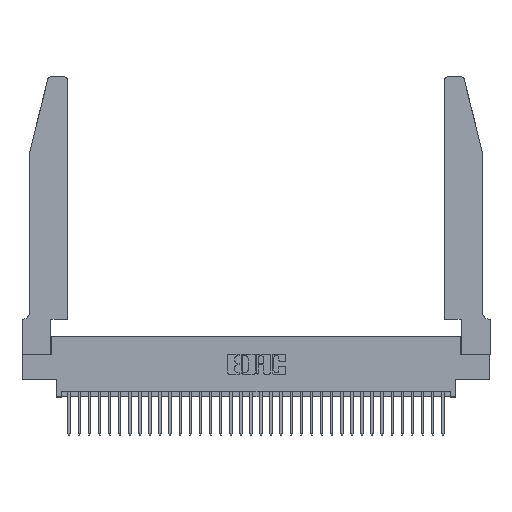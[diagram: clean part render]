
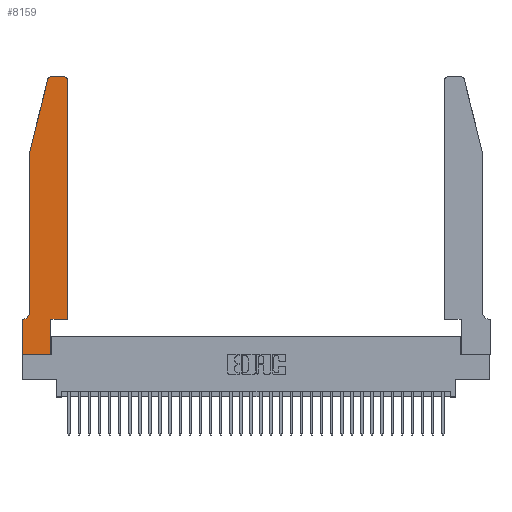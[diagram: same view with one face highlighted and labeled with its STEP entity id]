
A CAD part, top view. The second image highlights one B-rep face of the part: STEP entity #8159.
In plain terms, the highlighted planar face has unit normal (0, 0, 1).
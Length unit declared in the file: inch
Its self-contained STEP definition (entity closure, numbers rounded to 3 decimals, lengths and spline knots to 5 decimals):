
#110 = CARTESIAN_POINT ( 'NONE',  ( 0., 0., 0.37 ) ) ;
#474 = CIRCLE ( 'NONE', #28129, 0.03 ) ;
#939 = DIRECTION ( 'NONE',  ( 0., 0., 1. ) ) ;
#1340 = LINE ( 'NONE', #6033, #12000 ) ;
#2242 = EDGE_CURVE ( 'NONE', #10344, #26279, #31111, .T. ) ;
#2344 = DIRECTION ( 'NONE',  ( -1., 0., 0. ) ) ;
#3501 = VECTOR ( 'NONE', #15884, 39.37008 ) ;
#3804 = VECTOR ( 'NONE', #2344, 39.37008 ) ;
#4209 = ORIENTED_EDGE ( 'NONE', *, *, #34407, .T. ) ;
#4820 = AXIS2_PLACEMENT_3D ( 'NONE', #14662, #939, #14545 ) ;
#4962 = CARTESIAN_POINT ( 'NONE',  ( 0.4505, 0.35, 0.37 ) ) ;
#5090 = CARTESIAN_POINT ( 'NONE',  ( 0.4505, 2.72, 0.37 ) ) ;
#5333 = DIRECTION ( 'NONE',  ( 1., 0., 0. ) ) ;
#5356 = CARTESIAN_POINT ( 'NONE',  ( 0.4205, 2.75, 0.37 ) ) ;
#5872 = CARTESIAN_POINT ( 'NONE',  ( 0.284, 2.75, 0.37 ) ) ;
#6033 = CARTESIAN_POINT ( 'NONE',  ( 0.0755, 2., 0.37 ) ) ;
#6221 = VERTEX_POINT ( 'NONE', #25799 ) ;
#7044 = ORIENTED_EDGE ( 'NONE', *, *, #18117, .T. ) ;
#8021 = DIRECTION ( 'NONE',  ( 1., 0., 0. ) ) ;
#8159 = ADVANCED_FACE ( 'NONE', ( #14410 ), #26431, .T. ) ;
#8172 = VECTOR ( 'NONE', #12169, 39.37008 ) ;
#8259 = DIRECTION ( 'NONE',  ( 0., 0., -1. ) ) ;
#8478 = CARTESIAN_POINT ( 'NONE',  ( 0.4505, 0.35, 0.37 ) ) ;
#8535 = CARTESIAN_POINT ( 'NONE',  ( 0.25487, 2.72718, 0.37 ) ) ;
#9399 = VECTOR ( 'NONE', #11565, 39.37008 ) ;
#9536 = AXIS2_PLACEMENT_3D ( 'NONE', #21738, #8259, #18868 ) ;
#9808 = ORIENTED_EDGE ( 'NONE', *, *, #18643, .T. ) ;
#10032 = CARTESIAN_POINT ( 'NONE',  ( 0.0755, 2., 0.37 ) ) ;
#10326 = VECTOR ( 'NONE', #5333, 39.37008 ) ;
#10344 = VERTEX_POINT ( 'NONE', #28666 ) ;
#10536 = ORIENTED_EDGE ( 'NONE', *, *, #25302, .T. ) ;
#11201 = CARTESIAN_POINT ( 'NONE',  ( 0.2865, 0., 0.37 ) ) ;
#11354 = LINE ( 'NONE', #8478, #22037 ) ;
#11515 = DIRECTION ( 'NONE',  ( -0.239, -0.971, 0. ) ) ;
#11565 = DIRECTION ( 'NONE',  ( -1., 0., 0. ) ) ;
#11732 = VERTEX_POINT ( 'NONE', #8535 ) ;
#12000 = VECTOR ( 'NONE', #11515, 39.37008 ) ;
#12106 = EDGE_CURVE ( 'NONE', #34551, #10344, #24782, .T. ) ;
#12169 = DIRECTION ( 'NONE',  ( 0., 1., 0. ) ) ;
#12425 = EDGE_CURVE ( 'NONE', #18082, #6221, #20968, .T. ) ;
#12602 = CARTESIAN_POINT ( 'NONE',  ( 0.0755, 0.42, 0.37 ) ) ;
#13332 = LINE ( 'NONE', #10032, #3501 ) ;
#13388 = VECTOR ( 'NONE', #35286, 39.37008 ) ;
#13466 = EDGE_CURVE ( 'NONE', #31652, #23869, #15385, .T. ) ;
#14410 = FACE_OUTER_BOUND ( 'NONE', #34535, .T. ) ;
#14545 = DIRECTION ( 'NONE',  ( 1., 0., 0. ) ) ;
#14662 = CARTESIAN_POINT ( 'NONE',  ( 0.4205, 2.72, 0.37 ) ) ;
#15054 = CARTESIAN_POINT ( 'NONE',  ( 0.2865, 0.35, 0.37 ) ) ;
#15385 = LINE ( 'NONE', #18673, #3804 ) ;
#15562 = ORIENTED_EDGE ( 'NONE', *, *, #24809, .T. ) ;
#15884 = DIRECTION ( 'NONE',  ( 0., -1., 0. ) ) ;
#16419 = EDGE_CURVE ( 'NONE', #26704, #20437, #11354, .T. ) ;
#16990 = CARTESIAN_POINT ( 'NONE',  ( 0., 0.35, 0.37 ) ) ;
#17877 = ORIENTED_EDGE ( 'NONE', *, *, #18945, .T. ) ;
#18082 = VERTEX_POINT ( 'NONE', #11201 ) ;
#18117 = EDGE_CURVE ( 'NONE', #33977, #18082, #26115, .T. ) ;
#18242 = CARTESIAN_POINT ( 'NONE',  ( 0., 0., 0.37 ) ) ;
#18643 = EDGE_CURVE ( 'NONE', #6221, #26704, #35039, .T. ) ;
#18673 = CARTESIAN_POINT ( 'NONE',  ( 0.2605, 2.75, 0.37 ) ) ;
#18868 = DIRECTION ( 'NONE',  ( -1., 0., 0. ) ) ;
#18945 = EDGE_CURVE ( 'NONE', #11732, #25068, #1340, .T. ) ;
#20437 = VERTEX_POINT ( 'NONE', #5090 ) ;
#20585 = EDGE_CURVE ( 'NONE', #26279, #33977, #34033, .T. ) ;
#20915 = ORIENTED_EDGE ( 'NONE', *, *, #16419, .T. ) ;
#20968 = LINE ( 'NONE', #15054, #8172 ) ;
#21275 = VECTOR ( 'NONE', #24385, 39.37008 ) ;
#21600 = CARTESIAN_POINT ( 'NONE',  ( 0.4505, 0.35, 0.37 ) ) ;
#21738 = CARTESIAN_POINT ( 'NONE',  ( 0.0055, 0.42, 0.37 ) ) ;
#21834 = DIRECTION ( 'NONE',  ( 0., 0., 1. ) ) ;
#21940 = CARTESIAN_POINT ( 'NONE',  ( 0.0755, 2., 0.37 ) ) ;
#22037 = VECTOR ( 'NONE', #24637, 39.37008 ) ;
#23869 = VERTEX_POINT ( 'NONE', #5872 ) ;
#24159 = CARTESIAN_POINT ( 'NONE',  ( 0.284, 2.72, 0.37 ) ) ;
#24385 = DIRECTION ( 'NONE',  ( 0., -1., 0. ) ) ;
#24637 = DIRECTION ( 'NONE',  ( 0., 1., 0. ) ) ;
#24726 = ORIENTED_EDGE ( 'NONE', *, *, #12425, .T. ) ;
#24774 = CIRCLE ( 'NONE', #4820, 0.03 ) ;
#24782 = CIRCLE ( 'NONE', #9536, 0.07 ) ;
#24809 = EDGE_CURVE ( 'NONE', #25068, #34551, #13332, .T. ) ;
#25068 = VERTEX_POINT ( 'NONE', #21940 ) ;
#25302 = EDGE_CURVE ( 'NONE', #23869, #11732, #474, .T. ) ;
#25799 = CARTESIAN_POINT ( 'NONE',  ( 0.2865, 0.35, 0.37 ) ) ;
#26115 = LINE ( 'NONE', #32537, #13388 ) ;
#26279 = VERTEX_POINT ( 'NONE', #16990 ) ;
#26431 = PLANE ( 'NONE',  #34090 ) ;
#26704 = VERTEX_POINT ( 'NONE', #21600 ) ;
#27656 = ORIENTED_EDGE ( 'NONE', *, *, #12106, .T. ) ;
#27936 = ORIENTED_EDGE ( 'NONE', *, *, #2242, .T. ) ;
#28129 = AXIS2_PLACEMENT_3D ( 'NONE', #24159, #32137, #32380 ) ;
#28666 = CARTESIAN_POINT ( 'NONE',  ( 0.0055, 0.35, 0.37 ) ) ;
#28751 = ORIENTED_EDGE ( 'NONE', *, *, #20585, .T. ) ;
#31111 = LINE ( 'NONE', #33013, #9399 ) ;
#31652 = VERTEX_POINT ( 'NONE', #5356 ) ;
#32137 = DIRECTION ( 'NONE',  ( 0., 0., 1. ) ) ;
#32294 = CARTESIAN_POINT ( 'NONE',  ( 0., 0.35, 0.37 ) ) ;
#32380 = DIRECTION ( 'NONE',  ( 1., 0., 0. ) ) ;
#32537 = CARTESIAN_POINT ( 'NONE',  ( 0., 0., 0.37 ) ) ;
#33013 = CARTESIAN_POINT ( 'NONE',  ( 0.0755, 0.35, 0.37 ) ) ;
#33481 = ORIENTED_EDGE ( 'NONE', *, *, #13466, .T. ) ;
#33977 = VERTEX_POINT ( 'NONE', #18242 ) ;
#34033 = LINE ( 'NONE', #110, #21275 ) ;
#34090 = AXIS2_PLACEMENT_3D ( 'NONE', #32294, #21834, #8021 ) ;
#34407 = EDGE_CURVE ( 'NONE', #20437, #31652, #24774, .T. ) ;
#34535 = EDGE_LOOP ( 'NONE', ( #33481, #10536, #17877, #15562, #27656, #27936, #28751, #7044, #24726, #9808, #20915, #4209 ) ) ;
#34551 = VERTEX_POINT ( 'NONE', #12602 ) ;
#35039 = LINE ( 'NONE', #4962, #10326 ) ;
#35286 = DIRECTION ( 'NONE',  ( 1., 0., 0. ) ) ;
